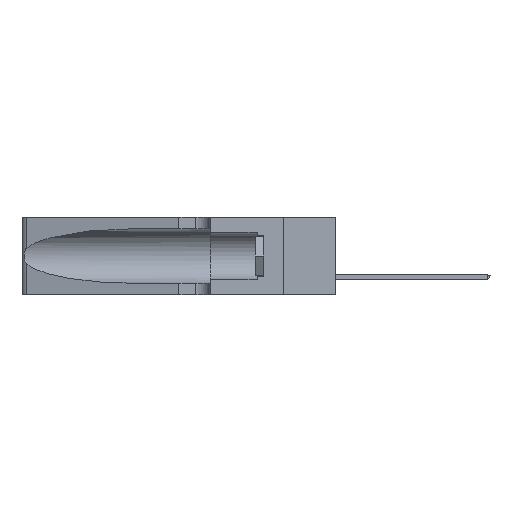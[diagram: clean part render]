
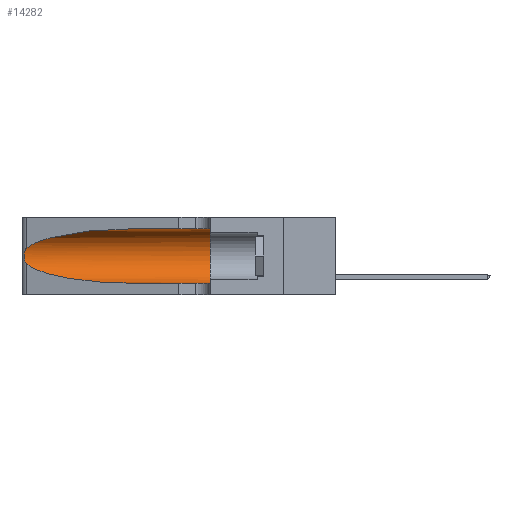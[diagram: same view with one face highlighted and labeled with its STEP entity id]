
A CAD part, left-side view. The second image highlights one B-rep face of the part: STEP entity #14282.
In plain terms, the highlighted cylindrical face has radius 3.308 mm (diameter 6.617 mm), a partial arc.
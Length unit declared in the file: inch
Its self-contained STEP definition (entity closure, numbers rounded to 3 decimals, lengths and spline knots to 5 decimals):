
#111 = CARTESIAN_POINT ( 'NONE',  ( 0.25487, 1.22718, 0.22369 ) ) ;
#802 = EDGE_CURVE ( 'NONE', #17536, #17418, #1370, .T. ) ;
#1270 = CARTESIAN_POINT ( 'NONE',  ( 0.25555, 1.22994, 0.2215 ) ) ;
#1357 = CARTESIAN_POINT ( 'NONE',  ( 0.25487, 1.22718, 0.14631 ) ) ;
#1370 = B_SPLINE_CURVE_WITH_KNOTS ( 'NONE', 3,
 ( #3012, #1270, #16987, #16828, #20790, #5250, #19078, #22646, #7174, #24633, #18815, #24907, #4908, #1357 ),
 .UNSPECIFIED., .F., .F.,
 ( 4, 2, 2, 2, 2, 2, 4 ),
 ( 0., 0.00027, 0.00053, 0.00107, 0.0016, 0.00187, 0.00214 ),
 .UNSPECIFIED. ) ;
#1536 = CARTESIAN_POINT ( 'NONE',  ( 0.1305, 0.72297, 0.31525 ) ) ;
#1652 = ORIENTED_EDGE ( 'NONE', *, *, #21316, .F. ) ;
#1831 = FACE_OUTER_BOUND ( 'NONE', #2284, .T. ) ;
#2209 = EDGE_CURVE ( 'NONE', #14970, #6640, #23612, .T. ) ;
#2284 = EDGE_LOOP ( 'NONE', ( #21418, #21016, #3251, #19711, #1652, #12090 ) ) ;
#3012 = CARTESIAN_POINT ( 'NONE',  ( 0.25487, 1.22718, 0.22369 ) ) ;
#3221 = VERTEX_POINT ( 'NONE', #19061 ) ;
#3251 = ORIENTED_EDGE ( 'NONE', *, *, #17079, .T. ) ;
#3550 = CARTESIAN_POINT ( 'NONE',  ( 0.25487, 1.22718, 0.22369 ) ) ;
#3740 = VERTEX_POINT ( 'NONE', #11686 ) ;
#4265 = CYLINDRICAL_SURFACE ( 'NONE', #7284, 0.13025 ) ;
#4908 = CARTESIAN_POINT ( 'NONE',  ( 0.25555, 1.22993, 0.14849 ) ) ;
#5250 = CARTESIAN_POINT ( 'NONE',  ( 0.26018, 1.23835, 0.19895 ) ) ;
#6107 = CIRCLE ( 'NONE', #6194, 0.13025 ) ;
#6194 = AXIS2_PLACEMENT_3D ( 'NONE', #20614, #8983, #12749 ) ;
#6298 = DIRECTION ( 'NONE',  ( 0., -1., 0. ) ) ;
#6640 = VERTEX_POINT ( 'NONE', #14634 ) ;
#6974 = VECTOR ( 'NONE', #6298, 39.37008 ) ;
#7174 = CARTESIAN_POINT ( 'NONE',  ( 0.26017, 1.23833, 0.17102 ) ) ;
#7270 = CARTESIAN_POINT ( 'NONE',  ( 0.18966, 0.96281, 0.31525 ) ) ;
#7284 = AXIS2_PLACEMENT_3D ( 'NONE', #14103, #16107, #18113 ) ;
#7893 =( BOUNDED_CURVE ( )  B_SPLINE_CURVE ( 3, ( #11249, #16902, #24808, #15228 ),
 .UNSPECIFIED., .F., .F. ) 
 B_SPLINE_CURVE_WITH_KNOTS ( ( 4, 4 ),
 ( 3.44316, 4.71239 ),
 .UNSPECIFIED. ) 
 CURVE ( )  GEOMETRIC_REPRESENTATION_ITEM ( )  RATIONAL_B_SPLINE_CURVE ( ( 1., 0.87, 0.87, 1. ) ) 
 REPRESENTATION_ITEM ( '' )  );
#8983 = DIRECTION ( 'NONE',  ( 0., 1., 0. ) ) ;
#11249 = CARTESIAN_POINT ( 'NONE',  ( 0.25487, 1.22718, 0.14631 ) ) ;
#11686 = CARTESIAN_POINT ( 'NONE',  ( 0.1305, 0.35, 0.05475 ) ) ;
#12090 = ORIENTED_EDGE ( 'NONE', *, *, #2209, .F. ) ;
#12248 = CARTESIAN_POINT ( 'NONE',  ( 0.1305, 1.61858, 0.31525 ) ) ;
#12456 =( BOUNDED_CURVE ( )  B_SPLINE_CURVE ( 3, ( #13296, #7270, #21063, #3550 ),
 .UNSPECIFIED., .F., .F. ) 
 B_SPLINE_CURVE_WITH_KNOTS ( ( 4, 4 ),
 ( 1.5708, 2.84003 ),
 .UNSPECIFIED. ) 
 CURVE ( )  GEOMETRIC_REPRESENTATION_ITEM ( )  RATIONAL_B_SPLINE_CURVE ( ( 1., 0.87, 0.87, 1. ) ) 
 REPRESENTATION_ITEM ( '' )  );
#12749 = DIRECTION ( 'NONE',  ( 0., 0., 1. ) ) ;
#13296 = CARTESIAN_POINT ( 'NONE',  ( 0.1305, 0.72297, 0.31525 ) ) ;
#13716 = VECTOR ( 'NONE', #25189, 39.37008 ) ;
#14103 = CARTESIAN_POINT ( 'NONE',  ( 0.1305, 1.61858, 0.185 ) ) ;
#14282 = ADVANCED_FACE ( 'NONE', ( #1831 ), #4265, .F. ) ;
#14634 = CARTESIAN_POINT ( 'NONE',  ( 0.1305, 0.35, 0.31525 ) ) ;
#14970 = VERTEX_POINT ( 'NONE', #1536 ) ;
#15228 = CARTESIAN_POINT ( 'NONE',  ( 0.1305, 0.72297, 0.05475 ) ) ;
#15974 = EDGE_CURVE ( 'NONE', #14970, #17536, #12456, .T. ) ;
#16107 = DIRECTION ( 'NONE',  ( 0., -1., 0. ) ) ;
#16828 = CARTESIAN_POINT ( 'NONE',  ( 0.25787, 1.23484, 0.2124 ) ) ;
#16902 = CARTESIAN_POINT ( 'NONE',  ( 0.2373, 1.15595, 0.08982 ) ) ;
#16987 = CARTESIAN_POINT ( 'NONE',  ( 0.25639, 1.23184, 0.21858 ) ) ;
#17079 = EDGE_CURVE ( 'NONE', #17418, #3221, #7893, .T. ) ;
#17418 = VERTEX_POINT ( 'NONE', #25493 ) ;
#17536 = VERTEX_POINT ( 'NONE', #111 ) ;
#17741 = LINE ( 'NONE', #21415, #13716 ) ;
#18113 = DIRECTION ( 'NONE',  ( 0., 0., -1. ) ) ;
#18815 = CARTESIAN_POINT ( 'NONE',  ( 0.25789, 1.23486, 0.15765 ) ) ;
#19061 = CARTESIAN_POINT ( 'NONE',  ( 0.1305, 0.72297, 0.05475 ) ) ;
#19078 = CARTESIAN_POINT ( 'NONE',  ( 0.26075, 1.23896, 0.19203 ) ) ;
#19711 = ORIENTED_EDGE ( 'NONE', *, *, #23787, .T. ) ;
#20614 = CARTESIAN_POINT ( 'NONE',  ( 0.1305, 0.35, 0.185 ) ) ;
#20790 = CARTESIAN_POINT ( 'NONE',  ( 0.25854, 1.2359, 0.20912 ) ) ;
#21016 = ORIENTED_EDGE ( 'NONE', *, *, #802, .T. ) ;
#21063 = CARTESIAN_POINT ( 'NONE',  ( 0.2373, 1.15595, 0.28018 ) ) ;
#21316 = EDGE_CURVE ( 'NONE', #6640, #3740, #6107, .T. ) ;
#21415 = CARTESIAN_POINT ( 'NONE',  ( 0.1305, 1.61858, 0.05475 ) ) ;
#21418 = ORIENTED_EDGE ( 'NONE', *, *, #15974, .T. ) ;
#22646 = CARTESIAN_POINT ( 'NONE',  ( 0.26075, 1.23896, 0.178 ) ) ;
#23612 = LINE ( 'NONE', #12248, #6974 ) ;
#23787 = EDGE_CURVE ( 'NONE', #3221, #3740, #17741, .T. ) ;
#24633 = CARTESIAN_POINT ( 'NONE',  ( 0.25856, 1.23593, 0.16098 ) ) ;
#24808 = CARTESIAN_POINT ( 'NONE',  ( 0.18966, 0.96281, 0.05475 ) ) ;
#24907 = CARTESIAN_POINT ( 'NONE',  ( 0.25639, 1.23186, 0.15144 ) ) ;
#25189 = DIRECTION ( 'NONE',  ( 0., -1., 0. ) ) ;
#25493 = CARTESIAN_POINT ( 'NONE',  ( 0.25487, 1.22718, 0.14631 ) ) ;
